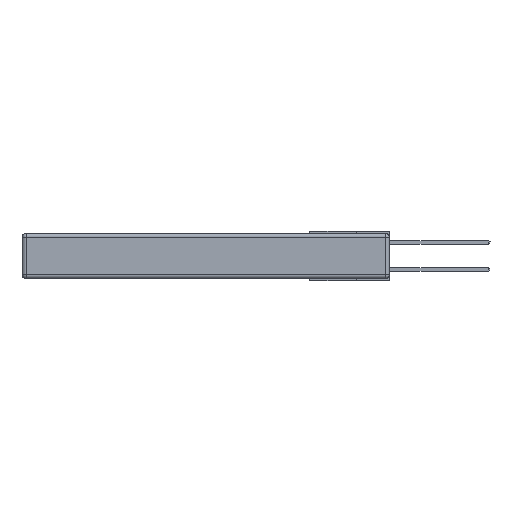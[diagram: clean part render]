
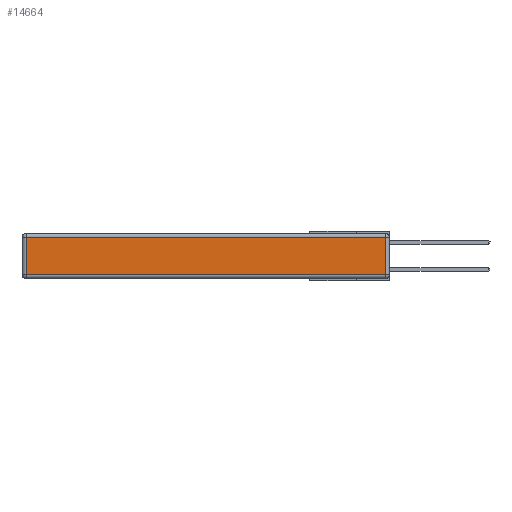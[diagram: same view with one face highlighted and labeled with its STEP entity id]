
A CAD part, left-side view. The second image highlights one B-rep face of the part: STEP entity #14664.
In plain terms, the highlighted planar face has unit normal (-1, 0, 0).
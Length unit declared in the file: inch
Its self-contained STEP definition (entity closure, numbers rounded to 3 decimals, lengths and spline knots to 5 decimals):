
#506 = DIRECTION ( 'NONE',  ( 0., 0., -1. ) ) ;
#579 = CARTESIAN_POINT ( 'NONE',  ( 0., 2.72, -0.313 ) ) ;
#1136 = CARTESIAN_POINT ( 'NONE',  ( 0., 0., -0.343 ) ) ;
#1409 = LINE ( 'NONE', #6952, #13422 ) ;
#1500 = VECTOR ( 'NONE', #10567, 39.37008 ) ;
#1662 = VECTOR ( 'NONE', #11987, 39.37008 ) ;
#2367 = EDGE_LOOP ( 'NONE', ( #9853, #5268, #11678, #13663 ) ) ;
#3318 = EDGE_CURVE ( 'NONE', #15577, #15317, #1409, .T. ) ;
#4103 = VERTEX_POINT ( 'NONE', #16295 ) ;
#4588 = AXIS2_PLACEMENT_3D ( 'NONE', #1136, #12614, #11129 ) ;
#5268 = ORIENTED_EDGE ( 'NONE', *, *, #15542, .T. ) ;
#5397 = DIRECTION ( 'NONE',  ( 0., -1., 0. ) ) ;
#6147 = CARTESIAN_POINT ( 'NONE',  ( 0., 2.75, -0.03 ) ) ;
#6613 = LINE ( 'NONE', #6147, #1500 ) ;
#6629 = EDGE_CURVE ( 'NONE', #9742, #4103, #6613, .T. ) ;
#6952 = CARTESIAN_POINT ( 'NONE',  ( 0., 0., -0.313 ) ) ;
#8274 = CARTESIAN_POINT ( 'NONE',  ( 0., 0.03, -0.03 ) ) ;
#9375 = LINE ( 'NONE', #17797, #12967 ) ;
#9742 = VERTEX_POINT ( 'NONE', #8274 ) ;
#9853 = ORIENTED_EDGE ( 'NONE', *, *, #3318, .T. ) ;
#9890 = LINE ( 'NONE', #10803, #1662 ) ;
#10446 = CARTESIAN_POINT ( 'NONE',  ( 0., 0.03, -0.313 ) ) ;
#10567 = DIRECTION ( 'NONE',  ( 0., 1., 0. ) ) ;
#10803 = CARTESIAN_POINT ( 'NONE',  ( 0., 0.03, -0.343 ) ) ;
#11129 = DIRECTION ( 'NONE',  ( 0., 0., 1. ) ) ;
#11678 = ORIENTED_EDGE ( 'NONE', *, *, #6629, .T. ) ;
#11987 = DIRECTION ( 'NONE',  ( 0., 0., 1. ) ) ;
#12614 = DIRECTION ( 'NONE',  ( -1., 0., 0. ) ) ;
#12967 = VECTOR ( 'NONE', #506, 39.37008 ) ;
#13422 = VECTOR ( 'NONE', #5397, 39.37008 ) ;
#13663 = ORIENTED_EDGE ( 'NONE', *, *, #17054, .T. ) ;
#14141 = PLANE ( 'NONE',  #4588 ) ;
#14664 = ADVANCED_FACE ( 'NONE', ( #14723 ), #14141, .T. ) ;
#14723 = FACE_OUTER_BOUND ( 'NONE', #2367, .T. ) ;
#15317 = VERTEX_POINT ( 'NONE', #10446 ) ;
#15542 = EDGE_CURVE ( 'NONE', #15317, #9742, #9890, .T. ) ;
#15577 = VERTEX_POINT ( 'NONE', #579 ) ;
#16295 = CARTESIAN_POINT ( 'NONE',  ( 0., 2.72, -0.03 ) ) ;
#17054 = EDGE_CURVE ( 'NONE', #4103, #15577, #9375, .T. ) ;
#17797 = CARTESIAN_POINT ( 'NONE',  ( 0., 2.72, -0.343 ) ) ;
